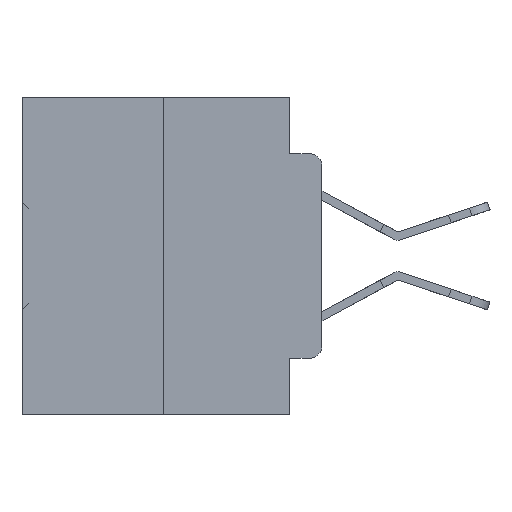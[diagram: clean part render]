
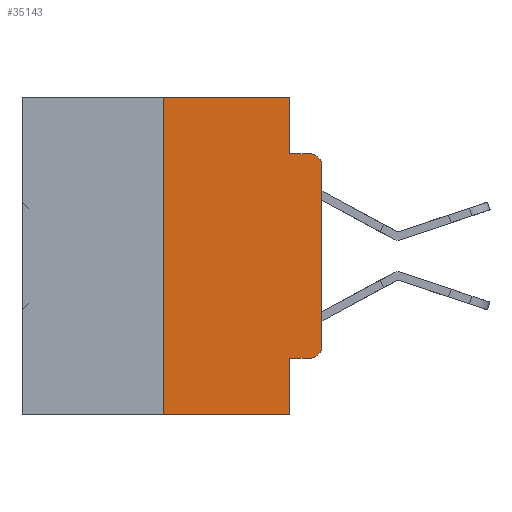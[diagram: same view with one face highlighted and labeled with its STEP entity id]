
A CAD part, left-side view. The second image highlights one B-rep face of the part: STEP entity #35143.
In plain terms, the highlighted planar face has unit normal (-1, 0, 0).
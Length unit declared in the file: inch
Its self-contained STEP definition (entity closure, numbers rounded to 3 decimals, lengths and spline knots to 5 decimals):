
#16 = EDGE_CURVE ( 'NONE', #29756, #7840, #36522, .T. ) ;
#797 = LINE ( 'NONE', #1617, #23780 ) ;
#1302 = DIRECTION ( 'NONE',  ( 0., 0., -1. ) ) ;
#1617 = CARTESIAN_POINT ( 'NONE',  ( 0., 0.25, 0. ) ) ;
#1755 = DIRECTION ( 'NONE',  ( 0., 0., 1. ) ) ;
#1894 = CARTESIAN_POINT ( 'NONE',  ( 0., 0.051, 0. ) ) ;
#2325 = EDGE_CURVE ( 'NONE', #11840, #16964, #12595, .T. ) ;
#3037 = ORIENTED_EDGE ( 'NONE', *, *, #31583, .T. ) ;
#3201 = VERTEX_POINT ( 'NONE', #32089 ) ;
#3389 = ORIENTED_EDGE ( 'NONE', *, *, #23631, .T. ) ;
#3989 = LINE ( 'NONE', #1894, #10990 ) ;
#4144 = VECTOR ( 'NONE', #32926, 39.37008 ) ;
#4900 = EDGE_CURVE ( 'NONE', #7902, #5503, #3989, .T. ) ;
#5142 = DIRECTION ( 'NONE',  ( 0., 0., 1. ) ) ;
#5503 = VERTEX_POINT ( 'NONE', #14317 ) ;
#6733 = DIRECTION ( 'NONE',  ( 1., 0., 0. ) ) ;
#7840 = VERTEX_POINT ( 'NONE', #12178 ) ;
#7902 = VERTEX_POINT ( 'NONE', #21457 ) ;
#8138 = CARTESIAN_POINT ( 'NONE',  ( 0., 0.02, -0.4115 ) ) ;
#9206 = DIRECTION ( 'NONE',  ( 0., -1., 0. ) ) ;
#10746 = AXIS2_PLACEMENT_3D ( 'NONE', #24591, #6733, #27578 ) ;
#10990 = VECTOR ( 'NONE', #1302, 39.37008 ) ;
#11174 = CARTESIAN_POINT ( 'NONE',  ( 0., 0.473, 0. ) ) ;
#11672 = CARTESIAN_POINT ( 'NONE',  ( 0., 0.02, -0.1085 ) ) ;
#11703 = ORIENTED_EDGE ( 'NONE', *, *, #2325, .F. ) ;
#11840 = VERTEX_POINT ( 'NONE', #37764 ) ;
#12178 = CARTESIAN_POINT ( 'NONE',  ( 0., 0.051, 0. ) ) ;
#12595 = LINE ( 'NONE', #29414, #27514 ) ;
#12600 = PLANE ( 'NONE',  #10746 ) ;
#12634 = VERTEX_POINT ( 'NONE', #26585 ) ;
#13386 = EDGE_CURVE ( 'NONE', #12634, #5503, #25229, .T. ) ;
#13418 = ORIENTED_EDGE ( 'NONE', *, *, #17429, .T. ) ;
#13617 = ORIENTED_EDGE ( 'NONE', *, *, #15331, .F. ) ;
#14317 = CARTESIAN_POINT ( 'NONE',  ( 0., 0.051, -0.5 ) ) ;
#14679 = DIRECTION ( 'NONE',  ( 0., 0., -1. ) ) ;
#15331 = EDGE_CURVE ( 'NONE', #7840, #11840, #27935, .T. ) ;
#16964 = VERTEX_POINT ( 'NONE', #21927 ) ;
#17141 = LINE ( 'NONE', #25833, #32029 ) ;
#17335 = VECTOR ( 'NONE', #29889, 39.37008 ) ;
#17429 = EDGE_CURVE ( 'NONE', #7902, #37633, #34286, .T. ) ;
#17968 = DIRECTION ( 'NONE',  ( -1., 0., 0. ) ) ;
#19304 = FACE_OUTER_BOUND ( 'NONE', #19644, .T. ) ;
#19644 = EDGE_LOOP ( 'NONE', ( #3037, #3389, #11703, #13617, #25244, #23688, #21111, #25641, #13418, #21348 ) ) ;
#19891 = VERTEX_POINT ( 'NONE', #29370 ) ;
#20802 = AXIS2_PLACEMENT_3D ( 'NONE', #35763, #17968, #38668 ) ;
#21111 = ORIENTED_EDGE ( 'NONE', *, *, #13386, .T. ) ;
#21348 = ORIENTED_EDGE ( 'NONE', *, *, #27378, .T. ) ;
#21457 = CARTESIAN_POINT ( 'NONE',  ( 0., 0.051, -0.4115 ) ) ;
#21645 = DIRECTION ( 'NONE',  ( 0., -1., 0. ) ) ;
#21927 = CARTESIAN_POINT ( 'NONE',  ( 0., 0.02, -0.0885 ) ) ;
#23631 = EDGE_CURVE ( 'NONE', #3201, #16964, #33625, .T. ) ;
#23688 = ORIENTED_EDGE ( 'NONE', *, *, #24589, .F. ) ;
#23780 = VECTOR ( 'NONE', #1755, 39.37008 ) ;
#24589 = EDGE_CURVE ( 'NONE', #12634, #29756, #797, .T. ) ;
#24591 = CARTESIAN_POINT ( 'NONE',  ( 0., 0.473, 0. ) ) ;
#25229 = LINE ( 'NONE', #32768, #17335 ) ;
#25244 = ORIENTED_EDGE ( 'NONE', *, *, #16, .F. ) ;
#25641 = ORIENTED_EDGE ( 'NONE', *, *, #4900, .F. ) ;
#25833 = CARTESIAN_POINT ( 'NONE',  ( 0., 0., 0. ) ) ;
#26585 = CARTESIAN_POINT ( 'NONE',  ( 0., 0.25, -0.5 ) ) ;
#27378 = EDGE_CURVE ( 'NONE', #37633, #19891, #30008, .T. ) ;
#27514 = VECTOR ( 'NONE', #29505, 39.37008 ) ;
#27578 = DIRECTION ( 'NONE',  ( 0., 0., -1. ) ) ;
#27598 = CARTESIAN_POINT ( 'NONE',  ( 0., 0.051, -0.4115 ) ) ;
#27935 = LINE ( 'NONE', #35911, #4144 ) ;
#28622 = VECTOR ( 'NONE', #9206, 39.37008 ) ;
#29370 = CARTESIAN_POINT ( 'NONE',  ( 0., 0., -0.3915 ) ) ;
#29414 = CARTESIAN_POINT ( 'NONE',  ( 0., 0.051, -0.0885 ) ) ;
#29505 = DIRECTION ( 'NONE',  ( 0., -1., 0. ) ) ;
#29756 = VERTEX_POINT ( 'NONE', #32845 ) ;
#29889 = DIRECTION ( 'NONE',  ( 0., -1., 0. ) ) ;
#30008 = CIRCLE ( 'NONE', #20802, 0.02 ) ;
#31583 = EDGE_CURVE ( 'NONE', #19891, #3201, #17141, .T. ) ;
#32029 = VECTOR ( 'NONE', #5142, 39.37008 ) ;
#32089 = CARTESIAN_POINT ( 'NONE',  ( 0., 0., -0.1085 ) ) ;
#32511 = DIRECTION ( 'NONE',  ( -1., 0., 0. ) ) ;
#32768 = CARTESIAN_POINT ( 'NONE',  ( 0., 0.473, -0.5 ) ) ;
#32845 = CARTESIAN_POINT ( 'NONE',  ( 0., 0.25, 0. ) ) ;
#32926 = DIRECTION ( 'NONE',  ( 0., 0., -1. ) ) ;
#33347 = VECTOR ( 'NONE', #21645, 39.37008 ) ;
#33625 = CIRCLE ( 'NONE', #38329, 0.02 ) ;
#34286 = LINE ( 'NONE', #27598, #33347 ) ;
#35143 = ADVANCED_FACE ( 'NONE', ( #19304 ), #12600, .F. ) ;
#35763 = CARTESIAN_POINT ( 'NONE',  ( 0., 0.02, -0.3915 ) ) ;
#35911 = CARTESIAN_POINT ( 'NONE',  ( 0., 0.051, 0. ) ) ;
#36522 = LINE ( 'NONE', #11174, #28622 ) ;
#37633 = VERTEX_POINT ( 'NONE', #8138 ) ;
#37764 = CARTESIAN_POINT ( 'NONE',  ( 0., 0.051, -0.0885 ) ) ;
#38329 = AXIS2_PLACEMENT_3D ( 'NONE', #11672, #32511, #14679 ) ;
#38668 = DIRECTION ( 'NONE',  ( 0., 0., -1. ) ) ;
